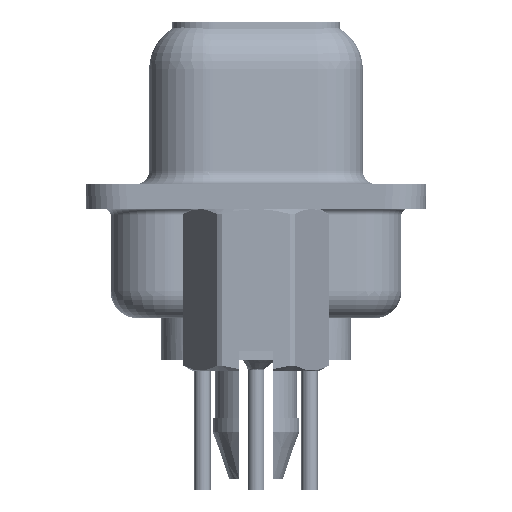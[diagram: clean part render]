
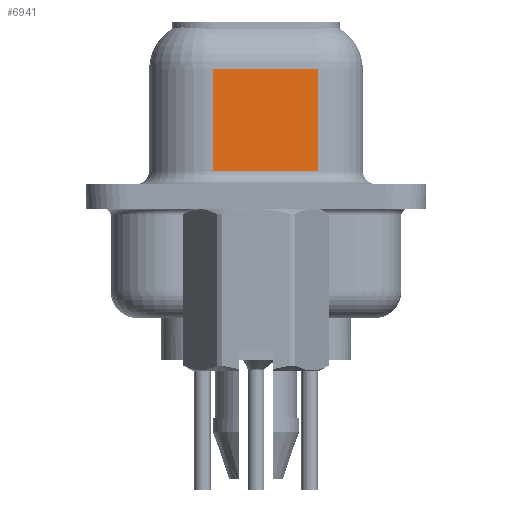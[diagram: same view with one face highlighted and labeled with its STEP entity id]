
A CAD part, left-side view. The second image highlights one B-rep face of the part: STEP entity #6941.
In plain terms, the highlighted planar face has unit normal (-0.985, -0.174, 0).
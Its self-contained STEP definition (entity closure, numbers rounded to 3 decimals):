
#685 = ORIENTED_EDGE ( 'NONE', *, *, #15560, .T. ) ;
#2086 = VECTOR ( 'NONE', #33713, 1000. ) ;
#2156 = CARTESIAN_POINT ( 'NONE',  ( 5.068, -2.297, 4.7 ) ) ;
#2218 = VECTOR ( 'NONE', #18429, 1000. ) ;
#3512 = ORIENTED_EDGE ( 'NONE', *, *, #7475, .T. ) ;
#6941 = ADVANCED_FACE ( 'NONE', ( #39090 ), #10310, .F. ) ;
#7434 = ORIENTED_EDGE ( 'NONE', *, *, #38912, .T. ) ;
#7475 = EDGE_CURVE ( 'NONE', #22822, #18724, #31474, .T. ) ;
#10310 = PLANE ( 'NONE',  #26159 ) ;
#11890 = VERTEX_POINT ( 'NONE', #31471 ) ;
#13184 = DIRECTION ( 'NONE',  ( 0.174, -0.985, 0. ) ) ;
#15560 = EDGE_CURVE ( 'NONE', #22192, #11890, #42922, .T. ) ;
#18429 = DIRECTION ( 'NONE',  ( 0., 0., -1. ) ) ;
#18724 = VERTEX_POINT ( 'NONE', #23189 ) ;
#19043 = CARTESIAN_POINT ( 'NONE',  ( 4.38, 1.603, 6.45 ) ) ;
#20273 = VECTOR ( 'NONE', #24092, 1000. ) ;
#22192 = VERTEX_POINT ( 'NONE', #44815 ) ;
#22822 = VERTEX_POINT ( 'NONE', #39254 ) ;
#23189 = CARTESIAN_POINT ( 'NONE',  ( 5.068, -2.297, 0.95 ) ) ;
#24092 = DIRECTION ( 'NONE',  ( -0.174, 0.985, 0. ) ) ;
#25158 = DIRECTION ( 'NONE',  ( 0.985, 0.174, 0. ) ) ;
#26159 = AXIS2_PLACEMENT_3D ( 'NONE', #39829, #25158, #32491 ) ;
#26701 = CARTESIAN_POINT ( 'NONE',  ( 5.068, -2.297, 6.45 ) ) ;
#29646 = LINE ( 'NONE', #26701, #2218 ) ;
#31471 = CARTESIAN_POINT ( 'NONE',  ( 4.38, 1.603, 4.7 ) ) ;
#31474 = LINE ( 'NONE', #31721, #42646 ) ;
#31721 = CARTESIAN_POINT ( 'NONE',  ( 5.068, -2.297, 0.95 ) ) ;
#32491 = DIRECTION ( 'NONE',  ( -0.174, 0.985, 0. ) ) ;
#33713 = DIRECTION ( 'NONE',  ( 0., 0., -1. ) ) ;
#34196 = LINE ( 'NONE', #19043, #2086 ) ;
#34512 = ORIENTED_EDGE ( 'NONE', *, *, #43828, .F. ) ;
#38912 = EDGE_CURVE ( 'NONE', #11890, #22822, #34196, .T. ) ;
#39090 = FACE_OUTER_BOUND ( 'NONE', #43281, .T. ) ;
#39254 = CARTESIAN_POINT ( 'NONE',  ( 4.38, 1.603, 0.95 ) ) ;
#39829 = CARTESIAN_POINT ( 'NONE',  ( 5.068, -2.297, 6.45 ) ) ;
#42646 = VECTOR ( 'NONE', #13184, 1000. ) ;
#42922 = LINE ( 'NONE', #2156, #20273 ) ;
#43281 = EDGE_LOOP ( 'NONE', ( #34512, #685, #7434, #3512 ) ) ;
#43828 = EDGE_CURVE ( 'NONE', #22192, #18724, #29646, .T. ) ;
#44815 = CARTESIAN_POINT ( 'NONE',  ( 5.068, -2.297, 4.7 ) ) ;
